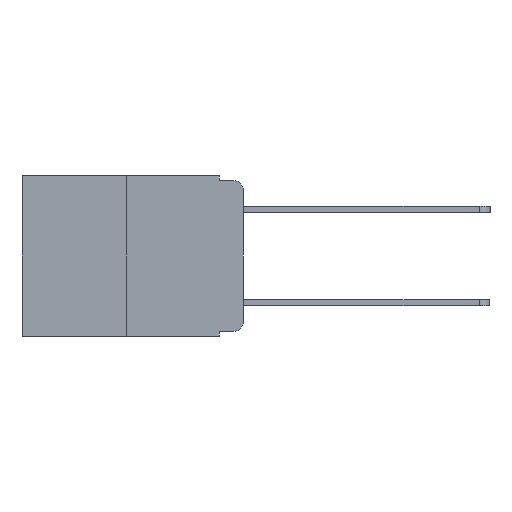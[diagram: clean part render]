
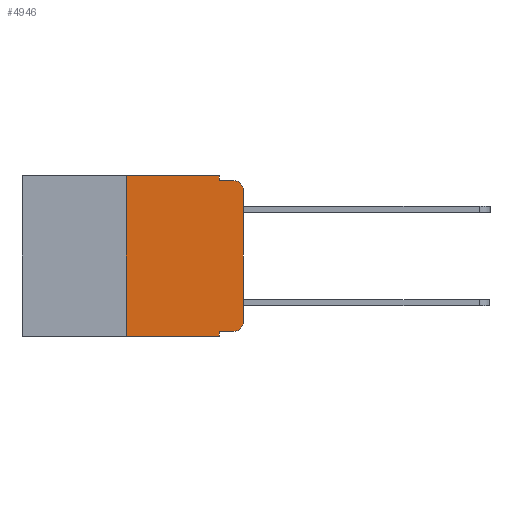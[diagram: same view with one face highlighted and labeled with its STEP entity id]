
A CAD part, left-side view. The second image highlights one B-rep face of the part: STEP entity #4946.
In plain terms, the highlighted planar face has unit normal (-1, 0, 0).
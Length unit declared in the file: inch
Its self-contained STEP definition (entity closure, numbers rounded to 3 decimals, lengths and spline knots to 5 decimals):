
#662 = VERTEX_POINT ( 'NONE', #9018 ) ;
#771 = AXIS2_PLACEMENT_3D ( 'NONE', #8235, #2098, #4928 ) ;
#1025 = LINE ( 'NONE', #10845, #10544 ) ;
#1131 = EDGE_CURVE ( 'NONE', #4256, #6883, #9256, .T. ) ;
#1180 = CIRCLE ( 'NONE', #7530, 0.02 ) ;
#1872 = LINE ( 'NONE', #10153, #6626 ) ;
#1881 = CARTESIAN_POINT ( 'NONE',  ( 0., 0.473, -0.343 ) ) ;
#1974 = DIRECTION ( 'NONE',  ( 0., 0., 1. ) ) ;
#2098 = DIRECTION ( 'NONE',  ( 1., 0., 0. ) ) ;
#2828 = AXIS2_PLACEMENT_3D ( 'NONE', #5289, #10869, #6262 ) ;
#2831 = EDGE_CURVE ( 'NONE', #662, #4193, #4425, .T. ) ;
#3134 = ORIENTED_EDGE ( 'NONE', *, *, #10073, .F. ) ;
#3149 = ORIENTED_EDGE ( 'NONE', *, *, #1131, .T. ) ;
#3164 = ORIENTED_EDGE ( 'NONE', *, *, #6878, .F. ) ;
#3181 = VERTEX_POINT ( 'NONE', #7269 ) ;
#3473 = EDGE_CURVE ( 'NONE', #3181, #4129, #3593, .T. ) ;
#3568 = DIRECTION ( 'NONE',  ( 0., -1., 0. ) ) ;
#3593 = LINE ( 'NONE', #5753, #5774 ) ;
#3836 = CARTESIAN_POINT ( 'NONE',  ( 0., 0.051, -0.343 ) ) ;
#3868 = LINE ( 'NONE', #8959, #9962 ) ;
#4013 = PLANE ( 'NONE',  #771 ) ;
#4129 = VERTEX_POINT ( 'NONE', #10324 ) ;
#4193 = VERTEX_POINT ( 'NONE', #8042 ) ;
#4256 = VERTEX_POINT ( 'NONE', #11173 ) ;
#4425 = LINE ( 'NONE', #10571, #8619 ) ;
#4493 = CARTESIAN_POINT ( 'NONE',  ( 0., 0.02, -0.03 ) ) ;
#4837 = CARTESIAN_POINT ( 'NONE',  ( 0., 0.051, 0. ) ) ;
#4928 = DIRECTION ( 'NONE',  ( 0., 0., -1. ) ) ;
#4946 = ADVANCED_FACE ( 'NONE', ( #11014 ), #4013, .F. ) ;
#5289 = CARTESIAN_POINT ( 'NONE',  ( 0., 0.02, -0.313 ) ) ;
#5460 = DIRECTION ( 'NONE',  ( 0., 0., -1. ) ) ;
#5753 = CARTESIAN_POINT ( 'NONE',  ( 0., 0., 0. ) ) ;
#5774 = VECTOR ( 'NONE', #1974, 39.37008 ) ;
#5878 = DIRECTION ( 'NONE',  ( 0., -1., 0. ) ) ;
#6059 = EDGE_LOOP ( 'NONE', ( #6581, #6108, #6296, #6312, #6483, #3164, #3149, #3134, #6198, #6511 ) ) ;
#6071 = VERTEX_POINT ( 'NONE', #8069 ) ;
#6108 = ORIENTED_EDGE ( 'NONE', *, *, #10601, .T. ) ;
#6198 = ORIENTED_EDGE ( 'NONE', *, *, #10545, .T. ) ;
#6235 = DIRECTION ( 'NONE',  ( 0., 0., -1. ) ) ;
#6262 = DIRECTION ( 'NONE',  ( 0., 0., -1. ) ) ;
#6296 = ORIENTED_EDGE ( 'NONE', *, *, #2831, .F. ) ;
#6312 = ORIENTED_EDGE ( 'NONE', *, *, #9606, .F. ) ;
#6350 = CARTESIAN_POINT ( 'NONE',  ( 0., 0.25, 0. ) ) ;
#6483 = ORIENTED_EDGE ( 'NONE', *, *, #9234, .F. ) ;
#6511 = ORIENTED_EDGE ( 'NONE', *, *, #10515, .T. ) ;
#6581 = ORIENTED_EDGE ( 'NONE', *, *, #3473, .T. ) ;
#6626 = VECTOR ( 'NONE', #10929, 39.37008 ) ;
#6878 = EDGE_CURVE ( 'NONE', #4256, #9765, #10111, .T. ) ;
#6883 = VERTEX_POINT ( 'NONE', #3836 ) ;
#7162 = CARTESIAN_POINT ( 'NONE',  ( 0., 0.02, -0.333 ) ) ;
#7234 = VECTOR ( 'NONE', #3568, 39.37008 ) ;
#7269 = CARTESIAN_POINT ( 'NONE',  ( 0., 0., -0.313 ) ) ;
#7530 = AXIS2_PLACEMENT_3D ( 'NONE', #4493, #10219, #5460 ) ;
#7814 = VECTOR ( 'NONE', #9680, 39.37008 ) ;
#7894 = VECTOR ( 'NONE', #10434, 39.37008 ) ;
#8042 = CARTESIAN_POINT ( 'NONE',  ( 0., 0.02, -0.01 ) ) ;
#8069 = CARTESIAN_POINT ( 'NONE',  ( 0., 0.051, -0.333 ) ) ;
#8235 = CARTESIAN_POINT ( 'NONE',  ( 0., 0.473, 0. ) ) ;
#8619 = VECTOR ( 'NONE', #5878, 39.37008 ) ;
#8761 = VERTEX_POINT ( 'NONE', #7162 ) ;
#8877 = CARTESIAN_POINT ( 'NONE',  ( 0., 0.25, 0. ) ) ;
#8959 = CARTESIAN_POINT ( 'NONE',  ( 0., 0.473, 0. ) ) ;
#9018 = CARTESIAN_POINT ( 'NONE',  ( 0., 0.051, -0.01 ) ) ;
#9234 = EDGE_CURVE ( 'NONE', #9765, #9252, #3868, .T. ) ;
#9252 = VERTEX_POINT ( 'NONE', #4837 ) ;
#9256 = LINE ( 'NONE', #1881, #7234 ) ;
#9606 = EDGE_CURVE ( 'NONE', #9252, #662, #1025, .T. ) ;
#9680 = DIRECTION ( 'NONE',  ( 0., 0., 1. ) ) ;
#9765 = VERTEX_POINT ( 'NONE', #6350 ) ;
#9827 = CIRCLE ( 'NONE', #2828, 0.02 ) ;
#9953 = LINE ( 'NONE', #11216, #7894 ) ;
#9962 = VECTOR ( 'NONE', #10503, 39.37008 ) ;
#10073 = EDGE_CURVE ( 'NONE', #6071, #6883, #9953, .T. ) ;
#10111 = LINE ( 'NONE', #8877, #7814 ) ;
#10153 = CARTESIAN_POINT ( 'NONE',  ( 0., 0.051, -0.333 ) ) ;
#10219 = DIRECTION ( 'NONE',  ( -1., 0., 0. ) ) ;
#10324 = CARTESIAN_POINT ( 'NONE',  ( 0., 0., -0.03 ) ) ;
#10434 = DIRECTION ( 'NONE',  ( 0., 0., -1. ) ) ;
#10503 = DIRECTION ( 'NONE',  ( 0., -1., 0. ) ) ;
#10515 = EDGE_CURVE ( 'NONE', #8761, #3181, #9827, .T. ) ;
#10544 = VECTOR ( 'NONE', #6235, 39.37008 ) ;
#10545 = EDGE_CURVE ( 'NONE', #6071, #8761, #1872, .T. ) ;
#10571 = CARTESIAN_POINT ( 'NONE',  ( 0., 0.051, -0.01 ) ) ;
#10601 = EDGE_CURVE ( 'NONE', #4129, #4193, #1180, .T. ) ;
#10845 = CARTESIAN_POINT ( 'NONE',  ( 0., 0.051, 0. ) ) ;
#10869 = DIRECTION ( 'NONE',  ( -1., 0., 0. ) ) ;
#10929 = DIRECTION ( 'NONE',  ( 0., -1., 0. ) ) ;
#11014 = FACE_OUTER_BOUND ( 'NONE', #6059, .T. ) ;
#11173 = CARTESIAN_POINT ( 'NONE',  ( 0., 0.25, -0.343 ) ) ;
#11216 = CARTESIAN_POINT ( 'NONE',  ( 0., 0.051, 0. ) ) ;
